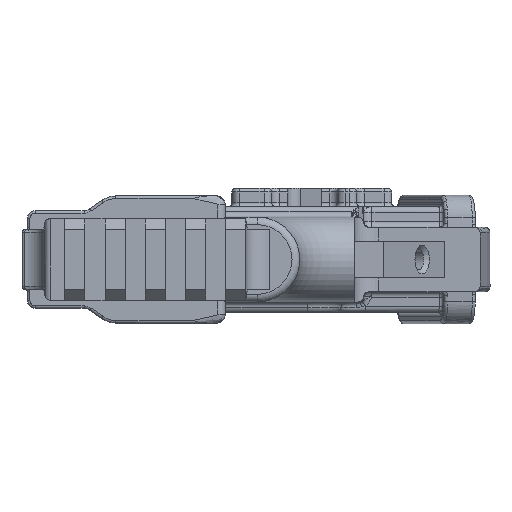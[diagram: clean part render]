
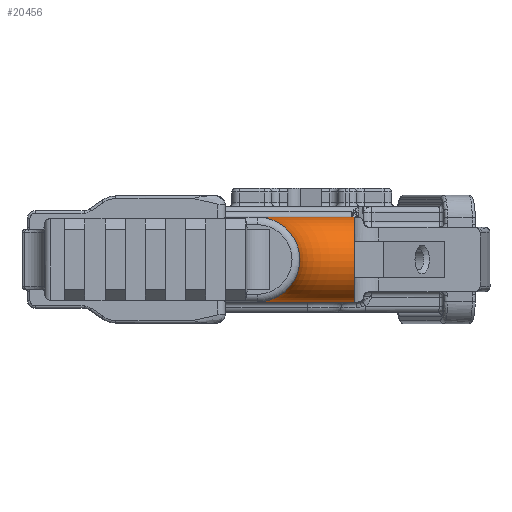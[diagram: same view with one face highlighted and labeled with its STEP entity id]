
A CAD part, left-side view. The second image highlights one B-rep face of the part: STEP entity #20456.
In plain terms, the highlighted toroidal (fillet/blend) face has major radius 30.1 mm and minor radius 11.05 mm.
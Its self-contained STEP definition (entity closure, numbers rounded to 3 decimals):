
#401=B_SPLINE_CURVE_WITH_KNOTS('',3,(#29287,#29288,#29289,#29290,#29291,
#29292,#29293,#29294,#29295,#29296,#29297,#29298,#29299,#29300,#29301,#29302,
#29303,#29304,#29305,#29306,#29307,#29308,#29309,#29310,#29311,#29312,#29313,
#29314,#29315,#29316,#29317,#29318,#29319,#29320),.UNSPECIFIED.,.F.,.F.,
(4,2,2,2,2,2,2,2,2,2,2,2,2,2,2,2,4),(-4.951,-4.742,
-4.533,-4.325,-4.116,-3.91,
-3.703,-3.501,-3.298,-3.095,
-2.892,-2.686,-2.48,-2.271,
-2.062,-1.854,-1.645),.UNSPECIFIED.);
#1670=TOROIDAL_SURFACE('',#21756,30.1,11.05);
#1804=FACE_OUTER_BOUND('',#2987,.T.);
#2987=EDGE_LOOP('',(#14426,#14427,#14428,#14429));
#8314=CIRCLE('',#21754,11.05);
#8315=CIRCLE('',#21757,30.1);
#8316=CIRCLE('',#21758,30.1);
#8989=VERTEX_POINT('',#29270);
#8990=VERTEX_POINT('',#29272);
#8995=VERTEX_POINT('',#29285);
#8996=VERTEX_POINT('',#29286);
#11100=EDGE_CURVE('',#8990,#8989,#8314,.T.);
#11106=EDGE_CURVE('',#8995,#8996,#401,.T.);
#11107=EDGE_CURVE('',#8990,#8996,#8315,.T.);
#11108=EDGE_CURVE('',#8989,#8995,#8316,.T.);
#14426=ORIENTED_EDGE('',*,*,#11106,.T.);
#14427=ORIENTED_EDGE('',*,*,#11107,.F.);
#14428=ORIENTED_EDGE('',*,*,#11100,.T.);
#14429=ORIENTED_EDGE('',*,*,#11108,.T.);
#20456=ADVANCED_FACE('',(#1804),#1670,.T.);
#21754=AXIS2_PLACEMENT_3D('',#29273,#23592,#23593);
#21756=AXIS2_PLACEMENT_3D('',#29284,#23601,#23602);
#21757=AXIS2_PLACEMENT_3D('',#29321,#23603,#23604);
#21758=AXIS2_PLACEMENT_3D('',#29322,#23605,#23606);
#23592=DIRECTION('center_axis',(1.,0.,0.));
#23593=DIRECTION('ref_axis',(0.,-0.233,-0.972));
#23601=DIRECTION('center_axis',(0.,0.,
-1.));
#23602=DIRECTION('ref_axis',(-1.,0.,0.));
#23603=DIRECTION('center_axis',(0.,0.,
-1.));
#23604=DIRECTION('ref_axis',(0.987,0.163,0.));
#23605=DIRECTION('center_axis',(0.,0.,
-1.));
#23606=DIRECTION('ref_axis',(0.987,0.163,0.));
#29270=CARTESIAN_POINT('',(-187.954,-1.95,-11.05));
#29272=CARTESIAN_POINT('',(-187.954,-1.95,11.05));
#29273=CARTESIAN_POINT('Origin',(-187.954,-1.95,0.));
#29284=CARTESIAN_POINT('Origin',(-187.954,-32.05,0.));
#29285=CARTESIAN_POINT('',(-158.256,-27.15,-11.05));
#29286=CARTESIAN_POINT('',(-158.256,-27.15,11.05));
#29287=CARTESIAN_POINT('Ctrl Pts',(-158.256,-27.15,-11.05));
#29288=CARTESIAN_POINT('Ctrl Pts',(-158.952,-27.15,-11.05));
#29289=CARTESIAN_POINT('Ctrl Pts',(-159.712,-27.15,-10.982));
#29290=CARTESIAN_POINT('Ctrl Pts',(-161.201,-27.15,-10.688));
#29291=CARTESIAN_POINT('Ctrl Pts',(-161.93,-27.15,-10.463));
#29292=CARTESIAN_POINT('Ctrl Pts',(-163.218,-27.15,-9.936));
#29293=CARTESIAN_POINT('Ctrl Pts',(-163.895,-27.15,-9.586));
#29294=CARTESIAN_POINT('Ctrl Pts',(-165.162,-27.15,-8.752));
#29295=CARTESIAN_POINT('Ctrl Pts',(-165.751,-27.15,-8.268));
#29296=CARTESIAN_POINT('Ctrl Pts',(-166.737,-27.15,-7.298));
#29297=CARTESIAN_POINT('Ctrl Pts',(-167.225,-27.15,-6.724));
#29298=CARTESIAN_POINT('Ctrl Pts',(-168.07,-27.15,-5.485));
#29299=CARTESIAN_POINT('Ctrl Pts',(-168.426,-27.15,-4.821));
#29300=CARTESIAN_POINT('Ctrl Pts',(-168.957,-27.15,-3.565));
#29301=CARTESIAN_POINT('Ctrl Pts',(-169.182,-27.15,-2.858));
#29302=CARTESIAN_POINT('Ctrl Pts',(-169.477,-27.15,-1.414));
#29303=CARTESIAN_POINT('Ctrl Pts',(-169.545,-27.15,-0.676));
#29304=CARTESIAN_POINT('Ctrl Pts',(-169.545,-27.15,0.676));
#29305=CARTESIAN_POINT('Ctrl Pts',(-169.477,-27.15,1.414));
#29306=CARTESIAN_POINT('Ctrl Pts',(-169.182,-27.15,2.858));
#29307=CARTESIAN_POINT('Ctrl Pts',(-168.957,-27.15,3.565));
#29308=CARTESIAN_POINT('Ctrl Pts',(-168.426,-27.15,4.821));
#29309=CARTESIAN_POINT('Ctrl Pts',(-168.07,-27.15,5.485));
#29310=CARTESIAN_POINT('Ctrl Pts',(-167.225,-27.15,6.724));
#29311=CARTESIAN_POINT('Ctrl Pts',(-166.737,-27.15,7.298));
#29312=CARTESIAN_POINT('Ctrl Pts',(-165.751,-27.15,8.268));
#29313=CARTESIAN_POINT('Ctrl Pts',(-165.162,-27.15,8.752));
#29314=CARTESIAN_POINT('Ctrl Pts',(-163.895,-27.15,9.586));
#29315=CARTESIAN_POINT('Ctrl Pts',(-163.218,-27.15,9.936));
#29316=CARTESIAN_POINT('Ctrl Pts',(-161.93,-27.15,10.463));
#29317=CARTESIAN_POINT('Ctrl Pts',(-161.201,-27.15,10.688));
#29318=CARTESIAN_POINT('Ctrl Pts',(-159.712,-27.15,10.982));
#29319=CARTESIAN_POINT('Ctrl Pts',(-158.952,-27.15,11.05));
#29320=CARTESIAN_POINT('Ctrl Pts',(-158.256,-27.15,11.05));
#29321=CARTESIAN_POINT('Origin',(-187.954,-32.05,11.05));
#29322=CARTESIAN_POINT('Origin',(-187.954,-32.05,-11.05));
